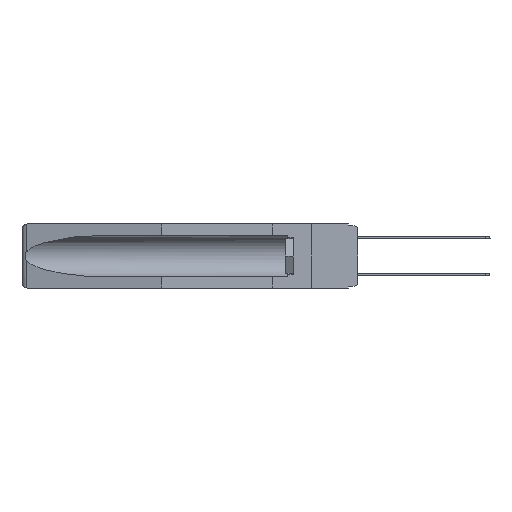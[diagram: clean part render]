
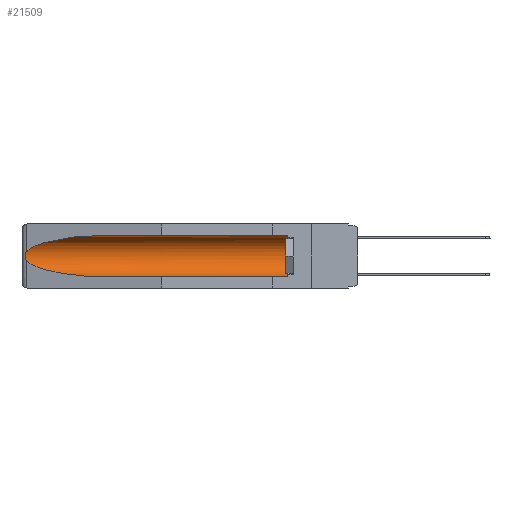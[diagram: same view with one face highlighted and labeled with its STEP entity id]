
A CAD part, left-side view. The second image highlights one B-rep face of the part: STEP entity #21509.
In plain terms, the highlighted cylindrical face has radius 2.857 mm (diameter 5.715 mm), a partial arc.
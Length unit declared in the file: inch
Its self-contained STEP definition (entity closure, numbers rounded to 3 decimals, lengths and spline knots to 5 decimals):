
#130 = DIRECTION ( 'NONE',  ( 0., 0., 1. ) ) ;
#151 = CARTESIAN_POINT ( 'NONE',  ( 0.155, 1.07973, -0.284 ) ) ;
#455 = CARTESIAN_POINT ( 'NONE',  ( 0.155, 1.07973, -0.059 ) ) ;
#475 = CARTESIAN_POINT ( 'NONE',  ( 0.25451, 1.48313, -0.09465 ) ) ;
#1138 = B_SPLINE_CURVE_WITH_KNOTS ( 'NONE', 3,
 ( #12886, #21778, #11183, #3935, #16328, #18087, #8103, #8029, #11420, #11502 ),
 .UNSPECIFIED., .F., .F.,
 ( 4, 2, 2, 2, 4 ),
 ( 0., 0.00029, 0.00058, 0.00087, 0.00117 ),
 .UNSPECIFIED. ) ;
#1423 =( BOUNDED_CURVE ( )  B_SPLINE_CURVE ( 3, ( #21353, #14067, #21119, #151 ),
 .UNSPECIFIED., .F., .T. ) 
 B_SPLINE_CURVE_WITH_KNOTS ( ( 4, 4 ),
 ( 0.1948, 1.5708 ),
 .UNSPECIFIED. ) 
 CURVE ( )  GEOMETRIC_REPRESENTATION_ITEM ( )  RATIONAL_B_SPLINE_CURVE ( ( 1., 0.848, 0.848, 1. ) ) 
 REPRESENTATION_ITEM ( '' )  );
#2279 = VERTEX_POINT ( 'NONE', #14317 ) ;
#3811 = CARTESIAN_POINT ( 'NONE',  ( 0.21114, 1.30732, -0.059 ) ) ;
#3935 = CARTESIAN_POINT ( 'NONE',  ( 0.2673, 1.5327, -0.16383 ) ) ;
#4428 = ORIENTED_EDGE ( 'NONE', *, *, #10828, .T. ) ;
#4755 = FACE_OUTER_BOUND ( 'NONE', #12473, .T. ) ;
#4960 = DIRECTION ( 'NONE',  ( 0., 0., 1. ) ) ;
#5759 = LINE ( 'NONE', #7001, #12419 ) ;
#7001 = CARTESIAN_POINT ( 'NONE',  ( 0.155, -0.30754, -0.059 ) ) ;
#7317 = VERTEX_POINT ( 'NONE', #455 ) ;
#8029 = CARTESIAN_POINT ( 'NONE',  ( 0.26655, 1.53094, -0.18657 ) ) ;
#8035 = CARTESIAN_POINT ( 'NONE',  ( 0.26537, 1.52718, -0.19328 ) ) ;
#8103 = CARTESIAN_POINT ( 'NONE',  ( 0.2673, 1.53269, -0.17917 ) ) ;
#8475 = VERTEX_POINT ( 'NONE', #13380 ) ;
#9057 = ORIENTED_EDGE ( 'NONE', *, *, #20375, .T. ) ;
#9178 = DIRECTION ( 'NONE',  ( 0., 1., 0. ) ) ;
#9340 =( BOUNDED_CURVE ( )  B_SPLINE_CURVE ( 3, ( #14612, #3811, #475, #12756 ),
 .UNSPECIFIED., .F., .T. ) 
 B_SPLINE_CURVE_WITH_KNOTS ( ( 4, 4 ),
 ( 4.71239, 6.08839 ),
 .UNSPECIFIED. ) 
 CURVE ( )  GEOMETRIC_REPRESENTATION_ITEM ( )  RATIONAL_B_SPLINE_CURVE ( ( 1., 0.848, 0.848, 1. ) ) 
 REPRESENTATION_ITEM ( '' )  );
#9720 = VERTEX_POINT ( 'NONE', #8035 ) ;
#10641 = VERTEX_POINT ( 'NONE', #13787 ) ;
#10713 = CARTESIAN_POINT ( 'NONE',  ( 0.155, 0.126, -0.059 ) ) ;
#10828 = EDGE_CURVE ( 'NONE', #7317, #8475, #9340, .T. ) ;
#11183 = CARTESIAN_POINT ( 'NONE',  ( 0.26654, 1.53092, -0.15636 ) ) ;
#11420 = CARTESIAN_POINT ( 'NONE',  ( 0.26597, 1.5296, -0.19026 ) ) ;
#11502 = CARTESIAN_POINT ( 'NONE',  ( 0.26537, 1.52718, -0.19328 ) ) ;
#12334 = ORIENTED_EDGE ( 'NONE', *, *, #22806, .T. ) ;
#12367 = EDGE_CURVE ( 'NONE', #22010, #7317, #5759, .T. ) ;
#12419 = VECTOR ( 'NONE', #21176, 39.37008 ) ;
#12461 = EDGE_CURVE ( 'NONE', #10641, #2279, #21525, .T. ) ;
#12473 = EDGE_LOOP ( 'NONE', ( #4428, #9057, #12334, #20336, #21386, #18049 ) ) ;
#12511 = CARTESIAN_POINT ( 'NONE',  ( 0.155, -0.30754, -0.1715 ) ) ;
#12756 = CARTESIAN_POINT ( 'NONE',  ( 0.26537, 1.52718, -0.14972 ) ) ;
#12886 = CARTESIAN_POINT ( 'NONE',  ( 0.26537, 1.52718, -0.14972 ) ) ;
#13380 = CARTESIAN_POINT ( 'NONE',  ( 0.26537, 1.52718, -0.14972 ) ) ;
#13787 = CARTESIAN_POINT ( 'NONE',  ( 0.155, 0.126, -0.284 ) ) ;
#14067 = CARTESIAN_POINT ( 'NONE',  ( 0.25451, 1.48313, -0.24835 ) ) ;
#14317 = CARTESIAN_POINT ( 'NONE',  ( 0.155, 1.07973, -0.284 ) ) ;
#14345 = DIRECTION ( 'NONE',  ( 0., 1., 0. ) ) ;
#14612 = CARTESIAN_POINT ( 'NONE',  ( 0.155, 1.07973, -0.059 ) ) ;
#15672 = AXIS2_PLACEMENT_3D ( 'NONE', #17169, #17252, #4960 ) ;
#16328 = CARTESIAN_POINT ( 'NONE',  ( 0.2675, 1.53308, -0.16763 ) ) ;
#16797 = EDGE_CURVE ( 'NONE', #10641, #22010, #19864, .T. ) ;
#16832 = VECTOR ( 'NONE', #9178, 39.37008 ) ;
#17023 = AXIS2_PLACEMENT_3D ( 'NONE', #12511, #14345, #130 ) ;
#17169 = CARTESIAN_POINT ( 'NONE',  ( 0.155, 0.126, -0.1715 ) ) ;
#17252 = DIRECTION ( 'NONE',  ( 0., -1., 0. ) ) ;
#17468 = CYLINDRICAL_SURFACE ( 'NONE', #17023, 0.1125 ) ;
#17999 = CARTESIAN_POINT ( 'NONE',  ( 0.155, -0.30754, -0.284 ) ) ;
#18049 = ORIENTED_EDGE ( 'NONE', *, *, #12367, .T. ) ;
#18087 = CARTESIAN_POINT ( 'NONE',  ( 0.2675, 1.53308, -0.17534 ) ) ;
#19864 = CIRCLE ( 'NONE', #15672, 0.1125 ) ;
#20336 = ORIENTED_EDGE ( 'NONE', *, *, #12461, .F. ) ;
#20375 = EDGE_CURVE ( 'NONE', #8475, #9720, #1138, .T. ) ;
#21119 = CARTESIAN_POINT ( 'NONE',  ( 0.21114, 1.30732, -0.284 ) ) ;
#21176 = DIRECTION ( 'NONE',  ( 0., 1., 0. ) ) ;
#21353 = CARTESIAN_POINT ( 'NONE',  ( 0.26537, 1.52718, -0.19328 ) ) ;
#21386 = ORIENTED_EDGE ( 'NONE', *, *, #16797, .T. ) ;
#21509 = ADVANCED_FACE ( 'NONE', ( #4755 ), #17468, .F. ) ;
#21525 = LINE ( 'NONE', #17999, #16832 ) ;
#21778 = CARTESIAN_POINT ( 'NONE',  ( 0.26597, 1.52961, -0.15275 ) ) ;
#22010 = VERTEX_POINT ( 'NONE', #10713 ) ;
#22806 = EDGE_CURVE ( 'NONE', #9720, #2279, #1423, .T. ) ;
